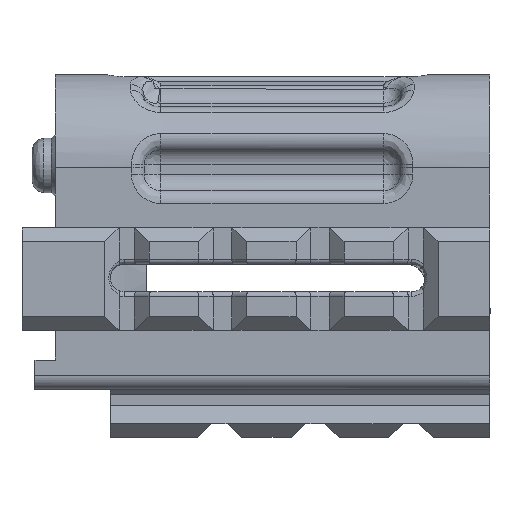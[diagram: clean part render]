
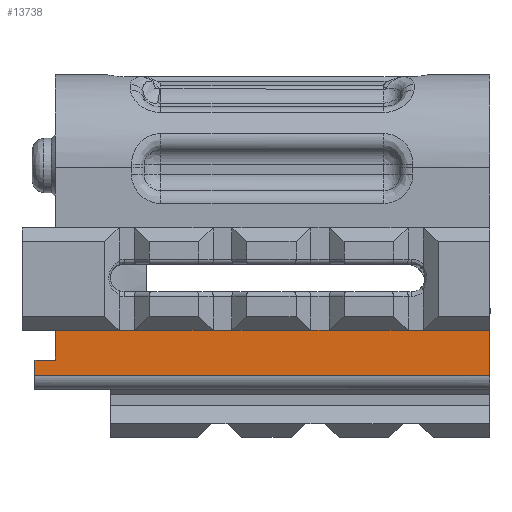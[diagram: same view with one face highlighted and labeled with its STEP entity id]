
A CAD part, top view. The second image highlights one B-rep face of the part: STEP entity #13738.
In plain terms, the highlighted planar face has unit normal (0, 0, 1).
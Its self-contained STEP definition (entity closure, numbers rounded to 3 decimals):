
#496 = VECTOR ( 'NONE', #12498, 1000. ) ;
#803 = EDGE_CURVE ( 'NONE', #11417, #10135, #11618, .T. ) ;
#910 = LINE ( 'NONE', #4267, #14592 ) ;
#1186 = CARTESIAN_POINT ( 'NONE',  ( 12.7, 6.41, 20.1 ) ) ;
#1198 = VERTEX_POINT ( 'NONE', #5035 ) ;
#1316 = EDGE_CURVE ( 'NONE', #10135, #2927, #910, .T. ) ;
#2102 = DIRECTION ( 'NONE',  ( 1., 0., 0. ) ) ;
#2498 = VECTOR ( 'NONE', #13442, 1000. ) ;
#2504 = ORIENTED_EDGE ( 'NONE', *, *, #1316, .T. ) ;
#2927 = VERTEX_POINT ( 'NONE', #7595 ) ;
#3794 = CARTESIAN_POINT ( 'NONE',  ( 12.7, 82.61, 20.1 ) ) ;
#3912 = CARTESIAN_POINT ( 'NONE',  ( 12.7, 15.707, 20.1 ) ) ;
#3943 = EDGE_CURVE ( 'NONE', #11651, #11417, #11767, .T. ) ;
#4257 = CARTESIAN_POINT ( 'NONE',  ( 12.7, 38.962, 20.1 ) ) ;
#4267 = CARTESIAN_POINT ( 'NONE',  ( 12.7, 3.06, 20.1 ) ) ;
#4799 = LINE ( 'NONE', #12036, #10151 ) ;
#4927 = EDGE_CURVE ( 'NONE', #2927, #1198, #4799, .T. ) ;
#5035 = CARTESIAN_POINT ( 'NONE',  ( 106.318, 15.707, 20.1 ) ) ;
#5172 = VECTOR ( 'NONE', #13750, 1000. ) ;
#5531 = VECTOR ( 'NONE', #10750, 1000. ) ;
#5686 = LINE ( 'NONE', #4257, #2498 ) ;
#6202 = CARTESIAN_POINT ( 'NONE',  ( 8.3, 82.61, 20.1 ) ) ;
#6222 = PLANE ( 'NONE',  #13346 ) ;
#6378 = DIRECTION ( 'NONE',  ( 0., 1., 0. ) ) ;
#6716 = LINE ( 'NONE', #11299, #496 ) ;
#7279 = DIRECTION ( 'NONE',  ( 0., -1., 0. ) ) ;
#7568 = ORIENTED_EDGE ( 'NONE', *, *, #3943, .T. ) ;
#7595 = CARTESIAN_POINT ( 'NONE',  ( 106.318, 3.06, 20.1 ) ) ;
#7674 = CARTESIAN_POINT ( 'NONE',  ( 12.7, 6.41, 20.1 ) ) ;
#7881 = EDGE_LOOP ( 'NONE', ( #2504, #12815, #9487, #12215, #7568, #13368 ) ) ;
#9487 = ORIENTED_EDGE ( 'NONE', *, *, #13214, .T. ) ;
#9912 = FACE_OUTER_BOUND ( 'NONE', #7881, .T. ) ;
#10062 = EDGE_CURVE ( 'NONE', #11651, #14191, #5686, .T. ) ;
#10135 = VERTEX_POINT ( 'NONE', #10198 ) ;
#10151 = VECTOR ( 'NONE', #6378, 1000. ) ;
#10198 = CARTESIAN_POINT ( 'NONE',  ( 8.3, 3.06, 20.1 ) ) ;
#10750 = DIRECTION ( 'NONE',  ( 0., -1., 0. ) ) ;
#11299 = CARTESIAN_POINT ( 'NONE',  ( 12.7, 15.707, 20.1 ) ) ;
#11417 = VERTEX_POINT ( 'NONE', #12953 ) ;
#11618 = LINE ( 'NONE', #6202, #5531 ) ;
#11651 = VERTEX_POINT ( 'NONE', #7674 ) ;
#11767 = LINE ( 'NONE', #1186, #5172 ) ;
#12036 = CARTESIAN_POINT ( 'NONE',  ( 106.318, 59.934, 20.1 ) ) ;
#12215 = ORIENTED_EDGE ( 'NONE', *, *, #10062, .F. ) ;
#12498 = DIRECTION ( 'NONE',  ( -1., 0., 0. ) ) ;
#12815 = ORIENTED_EDGE ( 'NONE', *, *, #4927, .T. ) ;
#12953 = CARTESIAN_POINT ( 'NONE',  ( 8.3, 6.41, 20.1 ) ) ;
#13214 = EDGE_CURVE ( 'NONE', #1198, #14191, #6716, .T. ) ;
#13346 = AXIS2_PLACEMENT_3D ( 'NONE', #3794, #14011, #7279 ) ;
#13368 = ORIENTED_EDGE ( 'NONE', *, *, #803, .T. ) ;
#13442 = DIRECTION ( 'NONE',  ( 0., 1., 0. ) ) ;
#13738 = ADVANCED_FACE ( 'NONE', ( #9912 ), #6222, .T. ) ;
#13750 = DIRECTION ( 'NONE',  ( -1., 0., 0. ) ) ;
#14011 = DIRECTION ( 'NONE',  ( 0., 0., 1. ) ) ;
#14191 = VERTEX_POINT ( 'NONE', #3912 ) ;
#14592 = VECTOR ( 'NONE', #2102, 1000. ) ;
